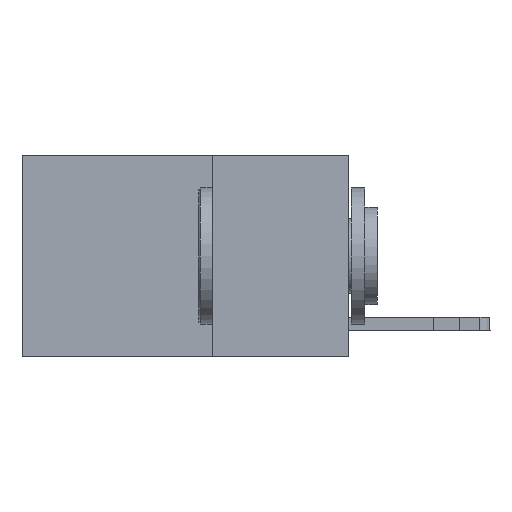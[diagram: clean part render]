
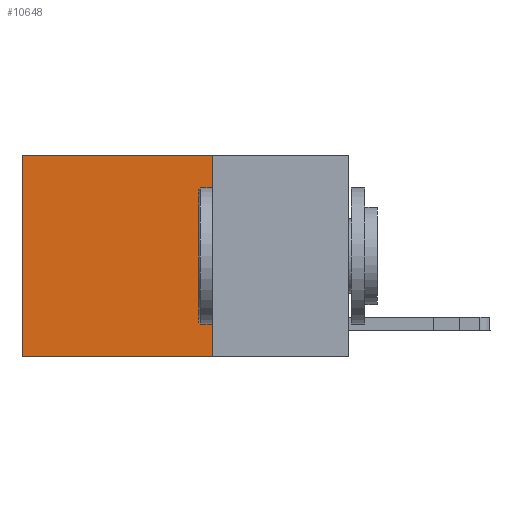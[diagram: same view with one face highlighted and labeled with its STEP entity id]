
A CAD part, left-side view. The second image highlights one B-rep face of the part: STEP entity #10648.
In plain terms, the highlighted planar face has unit normal (-1, 0, 0).
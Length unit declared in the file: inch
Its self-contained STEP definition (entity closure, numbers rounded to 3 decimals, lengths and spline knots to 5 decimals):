
#1231 = EDGE_CURVE ( 'NONE', #2122, #3569, #15595, .T. ) ;
#1721 = EDGE_CURVE ( 'NONE', #15536, #5776, #7700, .T. ) ;
#2027 = CARTESIAN_POINT ( 'NONE',  ( 0.2625, 0.25, 0. ) ) ;
#2122 = VERTEX_POINT ( 'NONE', #8168 ) ;
#2301 = VECTOR ( 'NONE', #11644, 39.37008 ) ;
#3149 = FACE_OUTER_BOUND ( 'NONE', #11258, .T. ) ;
#3427 = DIRECTION ( 'NONE',  ( 0., 0., -1. ) ) ;
#3569 = VERTEX_POINT ( 'NONE', #9269 ) ;
#3746 = DIRECTION ( 'NONE',  ( 0., 0., -1. ) ) ;
#3834 = LINE ( 'NONE', #16163, #4480 ) ;
#4480 = VECTOR ( 'NONE', #3746, 39.37008 ) ;
#4825 = DIRECTION ( 'NONE',  ( 0., 1., 0. ) ) ;
#5664 = ORIENTED_EDGE ( 'NONE', *, *, #16554, .T. ) ;
#5776 = VERTEX_POINT ( 'NONE', #13271 ) ;
#7484 = EDGE_CURVE ( 'NONE', #2122, #15536, #14614, .T. ) ;
#7685 = AXIS2_PLACEMENT_3D ( 'NONE', #11449, #14348, #14694 ) ;
#7700 = LINE ( 'NONE', #17557, #2301 ) ;
#7778 = CARTESIAN_POINT ( 'NONE',  ( 0.2625, 0.25, -0.37 ) ) ;
#8168 = CARTESIAN_POINT ( 'NONE',  ( 0.2625, 0.25, 0. ) ) ;
#9269 = CARTESIAN_POINT ( 'NONE',  ( 0.2625, 0.6, 0. ) ) ;
#9606 = VECTOR ( 'NONE', #3427, 39.37008 ) ;
#10431 = ORIENTED_EDGE ( 'NONE', *, *, #1231, .T. ) ;
#10648 = ADVANCED_FACE ( 'NONE', ( #3149 ), #16658, .F. ) ;
#10677 = ORIENTED_EDGE ( 'NONE', *, *, #7484, .F. ) ;
#11163 = ORIENTED_EDGE ( 'NONE', *, *, #1721, .F. ) ;
#11258 = EDGE_LOOP ( 'NONE', ( #5664, #11163, #10677, #10431 ) ) ;
#11449 = CARTESIAN_POINT ( 'NONE',  ( 0.2625, 0.25, 0. ) ) ;
#11644 = DIRECTION ( 'NONE',  ( 0., 1., 0. ) ) ;
#12974 = CARTESIAN_POINT ( 'NONE',  ( 0.2625, 0.25, 0. ) ) ;
#13271 = CARTESIAN_POINT ( 'NONE',  ( 0.2625, 0.6, -0.37 ) ) ;
#14348 = DIRECTION ( 'NONE',  ( 1., 0., 0. ) ) ;
#14489 = VECTOR ( 'NONE', #4825, 39.37008 ) ;
#14614 = LINE ( 'NONE', #12974, #9606 ) ;
#14694 = DIRECTION ( 'NONE',  ( 0., 0., -1. ) ) ;
#15536 = VERTEX_POINT ( 'NONE', #7778 ) ;
#15595 = LINE ( 'NONE', #2027, #14489 ) ;
#16163 = CARTESIAN_POINT ( 'NONE',  ( 0.2625, 0.6, 0. ) ) ;
#16554 = EDGE_CURVE ( 'NONE', #3569, #5776, #3834, .T. ) ;
#16658 = PLANE ( 'NONE',  #7685 ) ;
#17557 = CARTESIAN_POINT ( 'NONE',  ( 0.2625, 0.25, -0.37 ) ) ;
